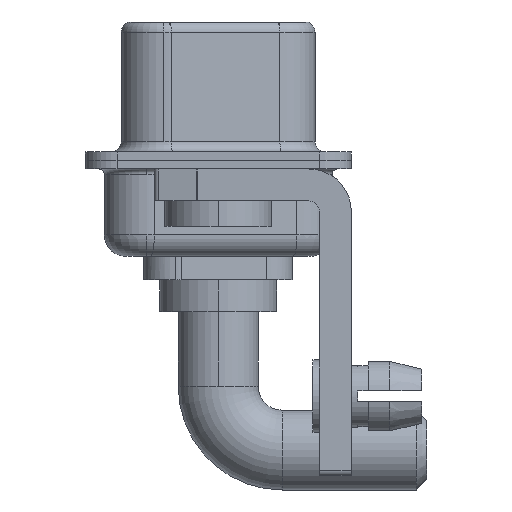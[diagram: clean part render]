
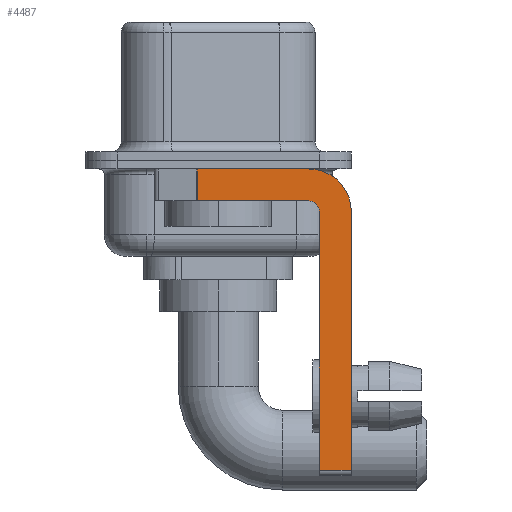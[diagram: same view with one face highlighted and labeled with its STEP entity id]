
A CAD part, left-side view. The second image highlights one B-rep face of the part: STEP entity #4487.
In plain terms, the highlighted planar face has unit normal (-1, 0, 0).
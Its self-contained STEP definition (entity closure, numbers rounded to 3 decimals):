
#141 = VECTOR ( 'NONE', #16016, 1000. ) ;
#194 = PLANE ( 'NONE',  #12971 ) ;
#381 = DIRECTION ( 'NONE',  ( 0., 0., -1. ) ) ;
#687 = VERTEX_POINT ( 'NONE', #5743 ) ;
#869 = ORIENTED_EDGE ( 'NONE', *, *, #2323, .T. ) ;
#891 = ORIENTED_EDGE ( 'NONE', *, *, #2649, .F. ) ;
#899 = CARTESIAN_POINT ( 'NONE',  ( -2.9, -6.25, -14.55 ) ) ;
#1003 = CARTESIAN_POINT ( 'NONE',  ( -2.9, -6.25, -2.4 ) ) ;
#1161 = DIRECTION ( 'NONE',  ( 0., 0., 1. ) ) ;
#1227 = AXIS2_PLACEMENT_3D ( 'NONE', #6828, #12393, #10881 ) ;
#1765 = DIRECTION ( 'NONE',  ( 0., 0., -1. ) ) ;
#1800 = DIRECTION ( 'NONE',  ( 1., 0., 0. ) ) ;
#2152 = VERTEX_POINT ( 'NONE', #12166 ) ;
#2181 = ORIENTED_EDGE ( 'NONE', *, *, #10246, .F. ) ;
#2272 = CARTESIAN_POINT ( 'NONE',  ( -2.9, -4.25, -1.9 ) ) ;
#2323 = EDGE_CURVE ( 'NONE', #687, #12402, #2636, .T. ) ;
#2627 = ORIENTED_EDGE ( 'NONE', *, *, #5677, .F. ) ;
#2636 = LINE ( 'NONE', #9633, #5279 ) ;
#2649 = EDGE_CURVE ( 'NONE', #10542, #12402, #4959, .T. ) ;
#2652 = CARTESIAN_POINT ( 'NONE',  ( -2.9, -4.75, -2.4 ) ) ;
#3696 = CARTESIAN_POINT ( 'NONE',  ( -2.9, 0.978, -0.4 ) ) ;
#3775 = DIRECTION ( 'NONE',  ( 0., 1., 0. ) ) ;
#3782 = CARTESIAN_POINT ( 'NONE',  ( -2.9, 0.978, -1.9 ) ) ;
#3964 = LINE ( 'NONE', #2272, #7874 ) ;
#4080 = LINE ( 'NONE', #15412, #18445 ) ;
#4111 = EDGE_CURVE ( 'NONE', #4882, #6363, #16909, .T. ) ;
#4145 = VECTOR ( 'NONE', #16499, 1000. ) ;
#4487 = ADVANCED_FACE ( 'NONE', ( #10293 ), #194, .F. ) ;
#4689 = EDGE_CURVE ( 'NONE', #6363, #9607, #3964, .T. ) ;
#4882 = VERTEX_POINT ( 'NONE', #2652 ) ;
#4959 = LINE ( 'NONE', #10723, #4145 ) ;
#5279 = VECTOR ( 'NONE', #8398, 1000. ) ;
#5677 = EDGE_CURVE ( 'NONE', #687, #4882, #4080, .T. ) ;
#5743 = CARTESIAN_POINT ( 'NONE',  ( -2.9, -4.75, -14.55 ) ) ;
#5948 = DIRECTION ( 'NONE',  ( 0., 0., -1. ) ) ;
#6363 = VERTEX_POINT ( 'NONE', #11129 ) ;
#6813 = EDGE_CURVE ( 'NONE', #2152, #10542, #15432, .T. ) ;
#6828 = CARTESIAN_POINT ( 'NONE',  ( -2.9, -4.25, -2.4 ) ) ;
#7630 = VECTOR ( 'NONE', #381, 1000. ) ;
#7874 = VECTOR ( 'NONE', #3775, 1000. ) ;
#8398 = DIRECTION ( 'NONE',  ( 0., -1., 0. ) ) ;
#8722 = CARTESIAN_POINT ( 'NONE',  ( -2.9, 0.978, -1.9 ) ) ;
#8760 = LINE ( 'NONE', #11855, #141 ) ;
#9607 = VERTEX_POINT ( 'NONE', #3782 ) ;
#9633 = CARTESIAN_POINT ( 'NONE',  ( -2.9, -4.25, -14.55 ) ) ;
#10246 = EDGE_CURVE ( 'NONE', #17896, #2152, #8760, .T. ) ;
#10293 = FACE_OUTER_BOUND ( 'NONE', #10911, .T. ) ;
#10528 = DIRECTION ( 'NONE',  ( 1., 0., 0. ) ) ;
#10542 = VERTEX_POINT ( 'NONE', #1003 ) ;
#10723 = CARTESIAN_POINT ( 'NONE',  ( -2.9, -6.25, -2.4 ) ) ;
#10881 = DIRECTION ( 'NONE',  ( 0., 0., 1. ) ) ;
#10911 = EDGE_LOOP ( 'NONE', ( #2181, #12849, #11892, #17965, #2627, #869, #891, #17425 ) ) ;
#11129 = CARTESIAN_POINT ( 'NONE',  ( -2.9, -4.25, -1.9 ) ) ;
#11855 = CARTESIAN_POINT ( 'NONE',  ( -2.9, 3., -0.4 ) ) ;
#11892 = ORIENTED_EDGE ( 'NONE', *, *, #4689, .F. ) ;
#12166 = CARTESIAN_POINT ( 'NONE',  ( -2.9, -4.25, -0.4 ) ) ;
#12393 = DIRECTION ( 'NONE',  ( -1., 0., 0. ) ) ;
#12402 = VERTEX_POINT ( 'NONE', #899 ) ;
#12849 = ORIENTED_EDGE ( 'NONE', *, *, #16485, .T. ) ;
#12971 = AXIS2_PLACEMENT_3D ( 'NONE', #14742, #1800, #5948 ) ;
#13313 = LINE ( 'NONE', #8722, #7630 ) ;
#13913 = AXIS2_PLACEMENT_3D ( 'NONE', #14704, #10528, #1765 ) ;
#14704 = CARTESIAN_POINT ( 'NONE',  ( -2.9, -4.25, -2.4 ) ) ;
#14742 = CARTESIAN_POINT ( 'NONE',  ( -2.9, -4.25, -2.4 ) ) ;
#15412 = CARTESIAN_POINT ( 'NONE',  ( -2.9, -4.75, -14.8 ) ) ;
#15432 = CIRCLE ( 'NONE', #13913, 2. ) ;
#16016 = DIRECTION ( 'NONE',  ( 0., -1., 0. ) ) ;
#16485 = EDGE_CURVE ( 'NONE', #17896, #9607, #13313, .T. ) ;
#16499 = DIRECTION ( 'NONE',  ( 0., 0., -1. ) ) ;
#16909 = CIRCLE ( 'NONE', #1227, 0.5 ) ;
#17425 = ORIENTED_EDGE ( 'NONE', *, *, #6813, .F. ) ;
#17896 = VERTEX_POINT ( 'NONE', #3696 ) ;
#17965 = ORIENTED_EDGE ( 'NONE', *, *, #4111, .F. ) ;
#18445 = VECTOR ( 'NONE', #1161, 1000. ) ;
